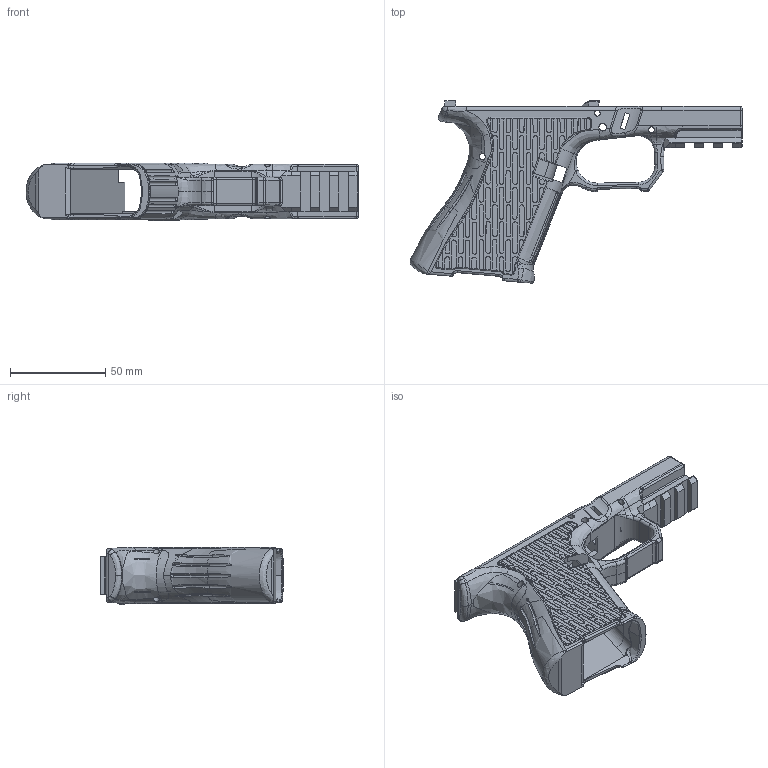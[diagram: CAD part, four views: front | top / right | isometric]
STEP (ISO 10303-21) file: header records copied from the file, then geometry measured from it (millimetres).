
FILE_DESCRIPTION(/* description */ (''),/* implementation_level */ '2;1');
FILE_NAME(/* name */ 'G26X Thicc.step',/* time_stamp */ '2022-07-20T09:54:50-06:00',/* author */ (''),/* organization */ (''),/* preprocessor_version */ 'ST-DEVELOPER v19',/* originating_system */ 'Autodesk Translation Framework v11.7.0.108',/* authorisation */ '');
FILE_SCHEMA (('AUTOMOTIVE_DESIGN { 1 0 10303 214 3 1 1 }'));
Products named in the file (1): G26X
Bounding box: 174.22 x 95.82 x 30.34 mm (x, y, z)
Volume: 88724.6 mm3; surface area: 45009.2 mm2
Topology: 1 solids, 1 shells, 2008 faces, 5545 edges, 3549 vertices
Faces by surface type: bspline 986, plane 685, cylinder 246, torus 68, sphere 18, cone 5
Full cylindrical faces by diameter (mm): 2 x1, 3 x4, 3.2 x2, 4 x2
Entity records: 96566 total; most frequent: CARTESIAN_POINT 54249, ORIENTED_EDGE 11066, DIRECTION 6255, EDGE_CURVE 5533, VERTEX_POINT 3550, LINE 2557, VECTOR 2557, EDGE_LOOP 2061
